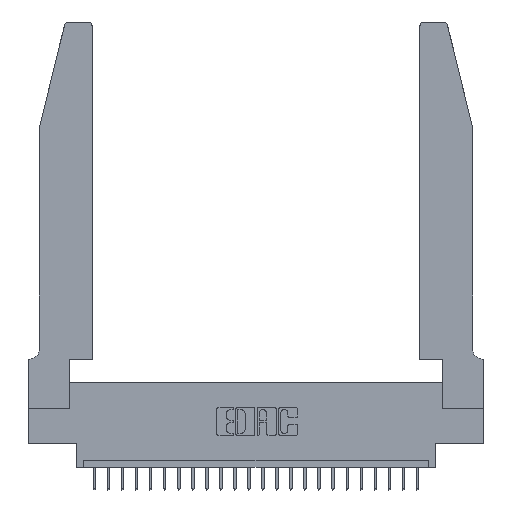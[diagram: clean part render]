
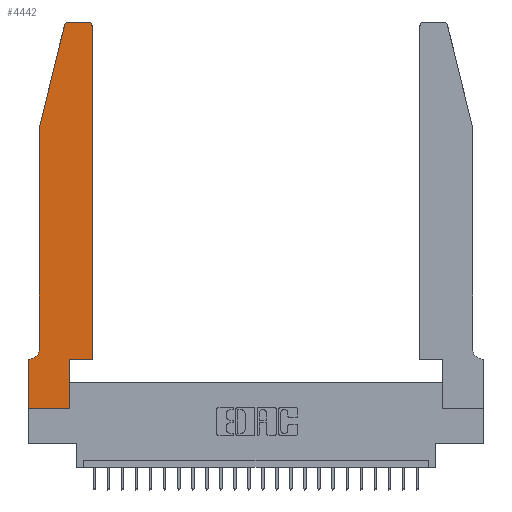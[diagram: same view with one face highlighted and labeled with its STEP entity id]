
A CAD part, top view. The second image highlights one B-rep face of the part: STEP entity #4442.
In plain terms, the highlighted planar face has unit normal (0, 0, 1).
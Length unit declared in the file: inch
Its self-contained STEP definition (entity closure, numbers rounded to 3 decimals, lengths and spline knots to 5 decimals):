
#165 = DIRECTION ( 'NONE',  ( 0., -1., 0. ) ) ;
#182 = DIRECTION ( 'NONE',  ( 0., 0., 1. ) ) ;
#469 = FACE_OUTER_BOUND ( 'NONE', #19559, .T. ) ;
#816 = DIRECTION ( 'NONE',  ( 0., 1., 0. ) ) ;
#1019 = CARTESIAN_POINT ( 'NONE',  ( 0.0755, 2., 0.37 ) ) ;
#1049 = LINE ( 'NONE', #18259, #2913 ) ;
#1362 = LINE ( 'NONE', #21757, #18263 ) ;
#1366 = CARTESIAN_POINT ( 'NONE',  ( 0.0055, 0.35, 0.37 ) ) ;
#1421 = VECTOR ( 'NONE', #18903, 39.37008 ) ;
#1800 = EDGE_CURVE ( 'NONE', #17597, #4335, #6121, .T. ) ;
#1900 = CARTESIAN_POINT ( 'NONE',  ( 0.4205, 2.72, 0.37 ) ) ;
#2124 = VERTEX_POINT ( 'NONE', #22242 ) ;
#2382 = CARTESIAN_POINT ( 'NONE',  ( 0.4505, 0.35, 0.37 ) ) ;
#2799 = ORIENTED_EDGE ( 'NONE', *, *, #12336, .T. ) ;
#2841 = CARTESIAN_POINT ( 'NONE',  ( 0.0755, 0.35, 0.37 ) ) ;
#2850 = CARTESIAN_POINT ( 'NONE',  ( 0.2865, 0., 0.37 ) ) ;
#2913 = VECTOR ( 'NONE', #10468, 39.37008 ) ;
#3314 = CARTESIAN_POINT ( 'NONE',  ( 0.0755, 2., 0.37 ) ) ;
#3324 = VERTEX_POINT ( 'NONE', #23824 ) ;
#3863 = EDGE_CURVE ( 'NONE', #12505, #3324, #24156, .T. ) ;
#4335 = VERTEX_POINT ( 'NONE', #12185 ) ;
#4442 = ADVANCED_FACE ( 'NONE', ( #469 ), #14758, .T. ) ;
#4642 = AXIS2_PLACEMENT_3D ( 'NONE', #20473, #18324, #14677 ) ;
#4668 = CARTESIAN_POINT ( 'NONE',  ( 0.0055, 0.42, 0.37 ) ) ;
#4689 = CARTESIAN_POINT ( 'NONE',  ( 0.2865, 0.35, 0.37 ) ) ;
#4706 = VECTOR ( 'NONE', #18619, 39.37008 ) ;
#5347 = ORIENTED_EDGE ( 'NONE', *, *, #11687, .T. ) ;
#5506 = EDGE_CURVE ( 'NONE', #3324, #25188, #20102, .T. ) ;
#5567 = EDGE_CURVE ( 'NONE', #14017, #12505, #19788, .T. ) ;
#5813 = ORIENTED_EDGE ( 'NONE', *, *, #13966, .T. ) ;
#6121 = CIRCLE ( 'NONE', #11355, 0.03 ) ;
#7578 = EDGE_CURVE ( 'NONE', #19360, #9719, #1362, .T. ) ;
#7876 = CARTESIAN_POINT ( 'NONE',  ( 0., 0., 0.37 ) ) ;
#7934 = DIRECTION ( 'NONE',  ( 0., 0., 1. ) ) ;
#8636 = DIRECTION ( 'NONE',  ( 0., 0., -1. ) ) ;
#9393 = VECTOR ( 'NONE', #10840, 39.37008 ) ;
#9719 = VERTEX_POINT ( 'NONE', #15741 ) ;
#10464 = DIRECTION ( 'NONE',  ( 0., 1., 0. ) ) ;
#10468 = DIRECTION ( 'NONE',  ( -1., 0., 0. ) ) ;
#10840 = DIRECTION ( 'NONE',  ( -1., 0., 0. ) ) ;
#11355 = AXIS2_PLACEMENT_3D ( 'NONE', #11988, #182, #19545 ) ;
#11687 = EDGE_CURVE ( 'NONE', #13625, #15284, #19876, .T. ) ;
#11907 = VECTOR ( 'NONE', #15111, 39.37008 ) ;
#11988 = CARTESIAN_POINT ( 'NONE',  ( 0.284, 2.72, 0.37 ) ) ;
#12185 = CARTESIAN_POINT ( 'NONE',  ( 0.25487, 2.72718, 0.37 ) ) ;
#12336 = EDGE_CURVE ( 'NONE', #25188, #2124, #14966, .T. ) ;
#12505 = VERTEX_POINT ( 'NONE', #14474 ) ;
#12582 = CARTESIAN_POINT ( 'NONE',  ( 0.4505, 2.72, 0.37 ) ) ;
#12765 = EDGE_CURVE ( 'NONE', #21572, #19360, #15554, .T. ) ;
#12812 = ORIENTED_EDGE ( 'NONE', *, *, #22370, .T. ) ;
#13172 = AXIS2_PLACEMENT_3D ( 'NONE', #1900, #7934, #13705 ) ;
#13625 = VERTEX_POINT ( 'NONE', #14103 ) ;
#13705 = DIRECTION ( 'NONE',  ( 1., 0., 0. ) ) ;
#13966 = EDGE_CURVE ( 'NONE', #9719, #14017, #15893, .T. ) ;
#14017 = VERTEX_POINT ( 'NONE', #2850 ) ;
#14103 = CARTESIAN_POINT ( 'NONE',  ( 0.0755, 2., 0.37 ) ) ;
#14474 = CARTESIAN_POINT ( 'NONE',  ( 0.2865, 0.35, 0.37 ) ) ;
#14677 = DIRECTION ( 'NONE',  ( 1., 0., 0. ) ) ;
#14758 = PLANE ( 'NONE',  #4642 ) ;
#14966 = CIRCLE ( 'NONE', #13172, 0.03 ) ;
#15111 = DIRECTION ( 'NONE',  ( 1., 0., 0. ) ) ;
#15284 = VERTEX_POINT ( 'NONE', #24911 ) ;
#15554 = LINE ( 'NONE', #2841, #9393 ) ;
#15741 = CARTESIAN_POINT ( 'NONE',  ( 0., 0., 0.37 ) ) ;
#15893 = LINE ( 'NONE', #7876, #1421 ) ;
#16935 = ORIENTED_EDGE ( 'NONE', *, *, #12765, .T. ) ;
#17302 = DIRECTION ( 'NONE',  ( 0., -1., 0. ) ) ;
#17597 = VERTEX_POINT ( 'NONE', #23309 ) ;
#17912 = LINE ( 'NONE', #1019, #4706 ) ;
#18259 = CARTESIAN_POINT ( 'NONE',  ( 0.2605, 2.75, 0.37 ) ) ;
#18263 = VECTOR ( 'NONE', #165, 39.37008 ) ;
#18324 = DIRECTION ( 'NONE',  ( 0., 0., 1. ) ) ;
#18617 = ORIENTED_EDGE ( 'NONE', *, *, #23056, .T. ) ;
#18619 = DIRECTION ( 'NONE',  ( -0.239, -0.971, 0. ) ) ;
#18903 = DIRECTION ( 'NONE',  ( 1., 0., 0. ) ) ;
#19181 = VECTOR ( 'NONE', #10464, 39.37008 ) ;
#19214 = AXIS2_PLACEMENT_3D ( 'NONE', #4668, #8636, #22690 ) ;
#19360 = VERTEX_POINT ( 'NONE', #23837 ) ;
#19545 = DIRECTION ( 'NONE',  ( 1., 0., 0. ) ) ;
#19559 = EDGE_LOOP ( 'NONE', ( #21345, #24565, #18617, #5347, #12812, #16935, #21858, #5813, #21762, #24883, #21902, #2799 ) ) ;
#19788 = LINE ( 'NONE', #4689, #23744 ) ;
#19876 = LINE ( 'NONE', #3314, #22946 ) ;
#20102 = LINE ( 'NONE', #2382, #19181 ) ;
#20473 = CARTESIAN_POINT ( 'NONE',  ( 0., 0.35, 0.37 ) ) ;
#21345 = ORIENTED_EDGE ( 'NONE', *, *, #21901, .T. ) ;
#21572 = VERTEX_POINT ( 'NONE', #1366 ) ;
#21757 = CARTESIAN_POINT ( 'NONE',  ( 0., 0., 0.37 ) ) ;
#21762 = ORIENTED_EDGE ( 'NONE', *, *, #5567, .T. ) ;
#21858 = ORIENTED_EDGE ( 'NONE', *, *, #7578, .T. ) ;
#21901 = EDGE_CURVE ( 'NONE', #2124, #17597, #1049, .T. ) ;
#21902 = ORIENTED_EDGE ( 'NONE', *, *, #5506, .T. ) ;
#22242 = CARTESIAN_POINT ( 'NONE',  ( 0.4205, 2.75, 0.37 ) ) ;
#22370 = EDGE_CURVE ( 'NONE', #15284, #21572, #22859, .T. ) ;
#22690 = DIRECTION ( 'NONE',  ( -1., 0., 0. ) ) ;
#22859 = CIRCLE ( 'NONE', #19214, 0.07 ) ;
#22946 = VECTOR ( 'NONE', #17302, 39.37008 ) ;
#23056 = EDGE_CURVE ( 'NONE', #4335, #13625, #17912, .T. ) ;
#23309 = CARTESIAN_POINT ( 'NONE',  ( 0.284, 2.75, 0.37 ) ) ;
#23744 = VECTOR ( 'NONE', #816, 39.37008 ) ;
#23824 = CARTESIAN_POINT ( 'NONE',  ( 0.4505, 0.35, 0.37 ) ) ;
#23837 = CARTESIAN_POINT ( 'NONE',  ( 0., 0.35, 0.37 ) ) ;
#24156 = LINE ( 'NONE', #24904, #11907 ) ;
#24565 = ORIENTED_EDGE ( 'NONE', *, *, #1800, .T. ) ;
#24883 = ORIENTED_EDGE ( 'NONE', *, *, #3863, .T. ) ;
#24904 = CARTESIAN_POINT ( 'NONE',  ( 0.4505, 0.35, 0.37 ) ) ;
#24911 = CARTESIAN_POINT ( 'NONE',  ( 0.0755, 0.42, 0.37 ) ) ;
#25188 = VERTEX_POINT ( 'NONE', #12582 ) ;
